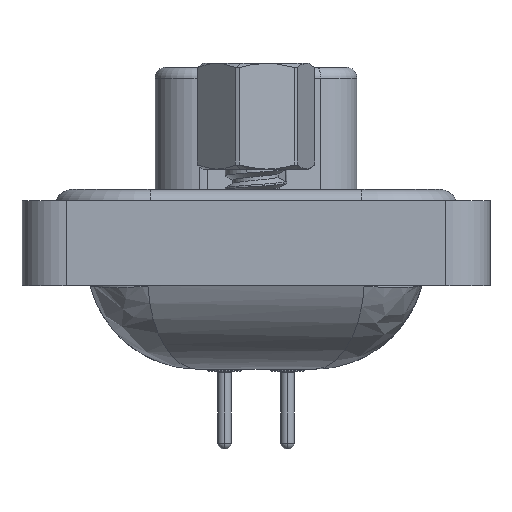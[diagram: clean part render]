
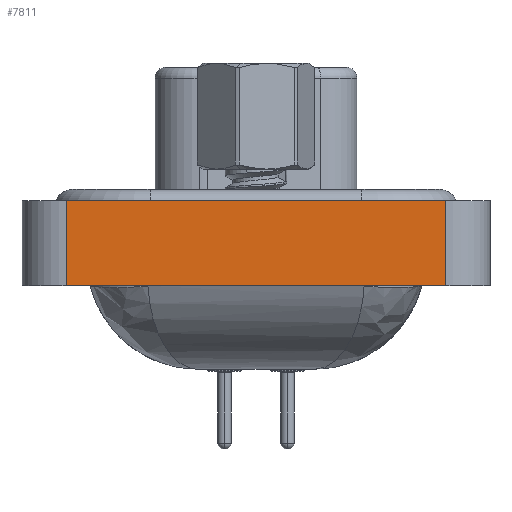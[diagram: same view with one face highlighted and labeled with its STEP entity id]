
A CAD part, left-side view. The second image highlights one B-rep face of the part: STEP entity #7811.
In plain terms, the highlighted planar face has unit normal (-1, 0, 0).
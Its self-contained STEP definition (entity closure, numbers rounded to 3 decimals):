
#540 = VERTEX_POINT ( 'NONE', #14021 ) ;
#710 = DIRECTION ( 'NONE',  ( -1., 0., 0. ) ) ;
#904 = AXIS2_PLACEMENT_3D ( 'NONE', #7039, #710, #14884 ) ;
#1146 = ORIENTED_EDGE ( 'NONE', *, *, #10817, .T. ) ;
#1989 = VERTEX_POINT ( 'NONE', #15461 ) ;
#3678 = ORIENTED_EDGE ( 'NONE', *, *, #5352, .F. ) ;
#3773 = VECTOR ( 'NONE', #9022, 1000. ) ;
#4103 = VERTEX_POINT ( 'NONE', #4432 ) ;
#4432 = CARTESIAN_POINT ( 'NONE',  ( -7.25, -8.55, 0.5 ) ) ;
#5352 = EDGE_CURVE ( 'NONE', #1989, #4103, #10972, .T. ) ;
#5410 = PLANE ( 'NONE',  #904 ) ;
#5458 = VECTOR ( 'NONE', #15011, 1000. ) ;
#5706 = VERTEX_POINT ( 'NONE', #9615 ) ;
#6188 = DIRECTION ( 'NONE',  ( 0., -1., 0. ) ) ;
#7039 = CARTESIAN_POINT ( 'NONE',  ( -7.25, -8.55, -3.35 ) ) ;
#7051 = VECTOR ( 'NONE', #6188, 1000. ) ;
#7270 = CARTESIAN_POINT ( 'NONE',  ( -7.25, -8.55, -3.35 ) ) ;
#7385 = CARTESIAN_POINT ( 'NONE',  ( -7.25, 8.55, -3.35 ) ) ;
#7520 = EDGE_CURVE ( 'NONE', #5706, #540, #13378, .T. ) ;
#7811 = ADVANCED_FACE ( 'NONE', ( #19466 ), #5410, .T. ) ;
#8808 = LINE ( 'NONE', #7385, #3773 ) ;
#9022 = DIRECTION ( 'NONE',  ( 0., 0., 1. ) ) ;
#9130 = ORIENTED_EDGE ( 'NONE', *, *, #7520, .T. ) ;
#9545 = CARTESIAN_POINT ( 'NONE',  ( -7.25, -8.55, 0.5 ) ) ;
#9615 = CARTESIAN_POINT ( 'NONE',  ( -7.25, 8.55, -3.35 ) ) ;
#9704 = LINE ( 'NONE', #14575, #15847 ) ;
#9961 = EDGE_CURVE ( 'NONE', #5706, #1989, #8808, .T. ) ;
#10817 = EDGE_CURVE ( 'NONE', #540, #4103, #9704, .T. ) ;
#10972 = LINE ( 'NONE', #9545, #7051 ) ;
#12673 = ORIENTED_EDGE ( 'NONE', *, *, #9961, .F. ) ;
#13378 = LINE ( 'NONE', #7270, #5458 ) ;
#14021 = CARTESIAN_POINT ( 'NONE',  ( -7.25, -8.55, -3.35 ) ) ;
#14575 = CARTESIAN_POINT ( 'NONE',  ( -7.25, -8.55, -3.35 ) ) ;
#14884 = DIRECTION ( 'NONE',  ( 0., 0., 1. ) ) ;
#15011 = DIRECTION ( 'NONE',  ( 0., -1., 0. ) ) ;
#15461 = CARTESIAN_POINT ( 'NONE',  ( -7.25, 8.55, 0.5 ) ) ;
#15847 = VECTOR ( 'NONE', #19255, 1000. ) ;
#19255 = DIRECTION ( 'NONE',  ( 0., 0., 1. ) ) ;
#19466 = FACE_OUTER_BOUND ( 'NONE', #19487, .T. ) ;
#19487 = EDGE_LOOP ( 'NONE', ( #1146, #3678, #12673, #9130 ) ) ;
